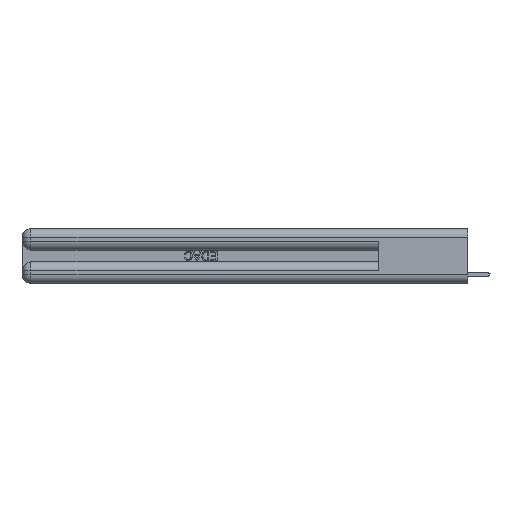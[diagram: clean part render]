
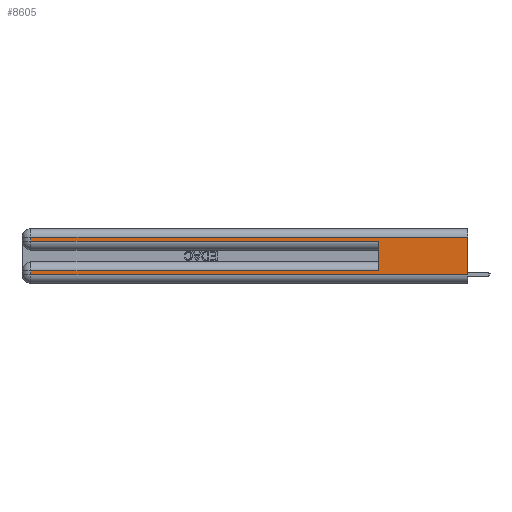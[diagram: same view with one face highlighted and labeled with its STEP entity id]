
A CAD part, left-side view. The second image highlights one B-rep face of the part: STEP entity #8605.
In plain terms, the highlighted planar face has unit normal (-1, 0, 0).
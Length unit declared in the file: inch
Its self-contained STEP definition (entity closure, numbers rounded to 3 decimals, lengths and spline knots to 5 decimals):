
#339 = VECTOR ( 'NONE', #13792, 39.37008 ) ;
#350 = EDGE_CURVE ( 'NONE', #24278, #18948, #4162, .T. ) ;
#802 = EDGE_LOOP ( 'NONE', ( #20792, #29832, #5039, #13038, #19828, #7912, #20027, #23296 ) ) ;
#1196 = CARTESIAN_POINT ( 'NONE',  ( 0., 2.94, 0.37 ) ) ;
#1959 = EDGE_CURVE ( 'NONE', #20688, #23185, #2638, .T. ) ;
#2638 = LINE ( 'NONE', #16141, #19085 ) ;
#3549 = EDGE_CURVE ( 'NONE', #23185, #26197, #22676, .T. ) ;
#4103 = CARTESIAN_POINT ( 'NONE',  ( 0., 0.6, 0.145 ) ) ;
#4162 = LINE ( 'NONE', #17531, #16663 ) ;
#4591 = CARTESIAN_POINT ( 'NONE',  ( 0., 2.94, 0.085 ) ) ;
#4615 = CARTESIAN_POINT ( 'NONE',  ( 0., 2.94, 0.37 ) ) ;
#4794 = EDGE_CURVE ( 'NONE', #20688, #16550, #25310, .T. ) ;
#5038 = PLANE ( 'NONE',  #25332 ) ;
#5039 = ORIENTED_EDGE ( 'NONE', *, *, #14211, .T. ) ;
#5463 = CARTESIAN_POINT ( 'NONE',  ( 0., 0.6, 0.085 ) ) ;
#6599 = CARTESIAN_POINT ( 'NONE',  ( 0., 2.94, 0.31 ) ) ;
#7411 = CARTESIAN_POINT ( 'NONE',  ( 0., 0., 0.285 ) ) ;
#7742 = CARTESIAN_POINT ( 'NONE',  ( 0., 2.94, 0.285 ) ) ;
#7912 = ORIENTED_EDGE ( 'NONE', *, *, #1959, .T. ) ;
#8605 = ADVANCED_FACE ( 'NONE', ( #19887 ), #5038, .F. ) ;
#8645 = VECTOR ( 'NONE', #26986, 39.37008 ) ;
#8843 = VECTOR ( 'NONE', #13075, 39.37008 ) ;
#9631 = DIRECTION ( 'NONE',  ( 1., 0., 0. ) ) ;
#10069 = LINE ( 'NONE', #22744, #8645 ) ;
#11763 = VECTOR ( 'NONE', #23414, 39.37008 ) ;
#11795 = VERTEX_POINT ( 'NONE', #6599 ) ;
#11899 = DIRECTION ( 'NONE',  ( 0., 0., -1. ) ) ;
#12916 = LINE ( 'NONE', #4615, #339 ) ;
#12990 = DIRECTION ( 'NONE',  ( 0., 0., -1. ) ) ;
#13038 = ORIENTED_EDGE ( 'NONE', *, *, #17993, .T. ) ;
#13075 = DIRECTION ( 'NONE',  ( 0., 0., 1. ) ) ;
#13792 = DIRECTION ( 'NONE',  ( 0., 0., -1. ) ) ;
#13826 = CARTESIAN_POINT ( 'NONE',  ( 0., 0., 0.06 ) ) ;
#14211 = EDGE_CURVE ( 'NONE', #11795, #21509, #12916, .T. ) ;
#15181 = LINE ( 'NONE', #18325, #28212 ) ;
#15277 = EDGE_CURVE ( 'NONE', #26197, #18948, #15181, .T. ) ;
#16141 = CARTESIAN_POINT ( 'NONE',  ( 0., 0., 0.085 ) ) ;
#16550 = VERTEX_POINT ( 'NONE', #20844 ) ;
#16663 = VECTOR ( 'NONE', #12990, 39.37008 ) ;
#16827 = EDGE_CURVE ( 'NONE', #24278, #11795, #10069, .T. ) ;
#17531 = CARTESIAN_POINT ( 'NONE',  ( 0., 0., 0.37 ) ) ;
#17993 = EDGE_CURVE ( 'NONE', #21509, #16550, #20034, .T. ) ;
#18325 = CARTESIAN_POINT ( 'NONE',  ( 0., 0., 0.06 ) ) ;
#18948 = VERTEX_POINT ( 'NONE', #13826 ) ;
#19085 = VECTOR ( 'NONE', #23372, 39.37008 ) ;
#19287 = DIRECTION ( 'NONE',  ( 0., -1., 0. ) ) ;
#19432 = VECTOR ( 'NONE', #26556, 39.37008 ) ;
#19828 = ORIENTED_EDGE ( 'NONE', *, *, #4794, .F. ) ;
#19887 = FACE_OUTER_BOUND ( 'NONE', #802, .T. ) ;
#20027 = ORIENTED_EDGE ( 'NONE', *, *, #3549, .T. ) ;
#20034 = LINE ( 'NONE', #7411, #11763 ) ;
#20688 = VERTEX_POINT ( 'NONE', #5463 ) ;
#20792 = ORIENTED_EDGE ( 'NONE', *, *, #350, .F. ) ;
#20844 = CARTESIAN_POINT ( 'NONE',  ( 0., 0.6, 0.285 ) ) ;
#21509 = VERTEX_POINT ( 'NONE', #7742 ) ;
#22112 = CARTESIAN_POINT ( 'NONE',  ( 0., 0., 0.31 ) ) ;
#22676 = LINE ( 'NONE', #1196, #19432 ) ;
#22744 = CARTESIAN_POINT ( 'NONE',  ( 0., 0., 0.31 ) ) ;
#23185 = VERTEX_POINT ( 'NONE', #4591 ) ;
#23296 = ORIENTED_EDGE ( 'NONE', *, *, #15277, .T. ) ;
#23346 = CARTESIAN_POINT ( 'NONE',  ( 0., 0., 0.37 ) ) ;
#23372 = DIRECTION ( 'NONE',  ( 0., 1., 0. ) ) ;
#23414 = DIRECTION ( 'NONE',  ( 0., -1., 0. ) ) ;
#24278 = VERTEX_POINT ( 'NONE', #22112 ) ;
#25310 = LINE ( 'NONE', #4103, #8843 ) ;
#25332 = AXIS2_PLACEMENT_3D ( 'NONE', #23346, #9631, #11899 ) ;
#26197 = VERTEX_POINT ( 'NONE', #28081 ) ;
#26556 = DIRECTION ( 'NONE',  ( 0., 0., -1. ) ) ;
#26986 = DIRECTION ( 'NONE',  ( 0., 1., 0. ) ) ;
#28081 = CARTESIAN_POINT ( 'NONE',  ( 0., 2.94, 0.06 ) ) ;
#28212 = VECTOR ( 'NONE', #19287, 39.37008 ) ;
#29832 = ORIENTED_EDGE ( 'NONE', *, *, #16827, .T. ) ;
